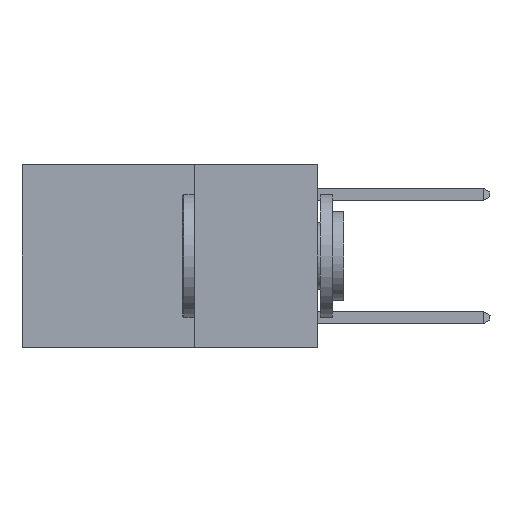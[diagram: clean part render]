
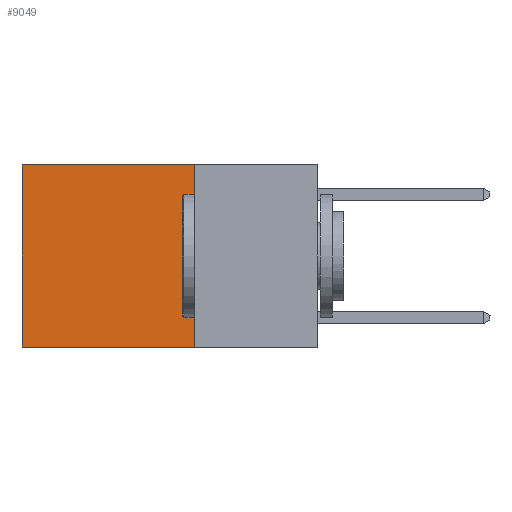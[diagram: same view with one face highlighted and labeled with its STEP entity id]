
A CAD part, left-side view. The second image highlights one B-rep face of the part: STEP entity #9049.
In plain terms, the highlighted planar face has unit normal (-1, 0, 0).
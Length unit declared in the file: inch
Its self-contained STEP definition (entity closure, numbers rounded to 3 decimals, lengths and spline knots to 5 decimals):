
#47 = EDGE_CURVE ( 'NONE', #16035, #13209, #1146, .T. ) ;
#61 = VERTEX_POINT ( 'NONE', #4878 ) ;
#372 = VECTOR ( 'NONE', #10680, 39.37008 ) ;
#576 = CARTESIAN_POINT ( 'NONE',  ( 0.2625, 0.25, 0. ) ) ;
#1146 = LINE ( 'NONE', #1954, #372 ) ;
#1410 = VECTOR ( 'NONE', #9944, 39.37008 ) ;
#1663 = DIRECTION ( 'NONE',  ( 0., 0., -1. ) ) ;
#1954 = CARTESIAN_POINT ( 'NONE',  ( 0.2625, 0.6, 0. ) ) ;
#2004 = LINE ( 'NONE', #16172, #1410 ) ;
#2369 = LINE ( 'NONE', #576, #11918 ) ;
#2755 = EDGE_LOOP ( 'NONE', ( #10230, #3491, #10836, #15406 ) ) ;
#2756 = LINE ( 'NONE', #13237, #7437 ) ;
#3491 = ORIENTED_EDGE ( 'NONE', *, *, #15170, .F. ) ;
#3964 = CARTESIAN_POINT ( 'NONE',  ( 0.2625, 0.6, -0.37 ) ) ;
#4878 = CARTESIAN_POINT ( 'NONE',  ( 0.2625, 0.25, -0.37 ) ) ;
#5680 = DIRECTION ( 'NONE',  ( 0., 0., -1. ) ) ;
#6031 = EDGE_CURVE ( 'NONE', #15231, #61, #2369, .T. ) ;
#6046 = EDGE_CURVE ( 'NONE', #15231, #16035, #2756, .T. ) ;
#7437 = VECTOR ( 'NONE', #13021, 39.37008 ) ;
#8159 = FACE_OUTER_BOUND ( 'NONE', #2755, .T. ) ;
#8835 = CARTESIAN_POINT ( 'NONE',  ( 0.2625, 0.25, 0. ) ) ;
#9049 = ADVANCED_FACE ( 'NONE', ( #8159 ), #15254, .F. ) ;
#9107 = CARTESIAN_POINT ( 'NONE',  ( 0.2625, 0.25, 0. ) ) ;
#9944 = DIRECTION ( 'NONE',  ( 0., 1., 0. ) ) ;
#10230 = ORIENTED_EDGE ( 'NONE', *, *, #47, .T. ) ;
#10680 = DIRECTION ( 'NONE',  ( 0., 0., -1. ) ) ;
#10836 = ORIENTED_EDGE ( 'NONE', *, *, #6031, .F. ) ;
#11225 = AXIS2_PLACEMENT_3D ( 'NONE', #9107, #12790, #1663 ) ;
#11918 = VECTOR ( 'NONE', #5680, 39.37008 ) ;
#12790 = DIRECTION ( 'NONE',  ( 1., 0., 0. ) ) ;
#13021 = DIRECTION ( 'NONE',  ( 0., 1., 0. ) ) ;
#13209 = VERTEX_POINT ( 'NONE', #3964 ) ;
#13237 = CARTESIAN_POINT ( 'NONE',  ( 0.2625, 0.25, 0. ) ) ;
#15170 = EDGE_CURVE ( 'NONE', #61, #13209, #2004, .T. ) ;
#15231 = VERTEX_POINT ( 'NONE', #8835 ) ;
#15254 = PLANE ( 'NONE',  #11225 ) ;
#15406 = ORIENTED_EDGE ( 'NONE', *, *, #6046, .T. ) ;
#16035 = VERTEX_POINT ( 'NONE', #16140 ) ;
#16140 = CARTESIAN_POINT ( 'NONE',  ( 0.2625, 0.6, 0. ) ) ;
#16172 = CARTESIAN_POINT ( 'NONE',  ( 0.2625, 0.25, -0.37 ) ) ;
